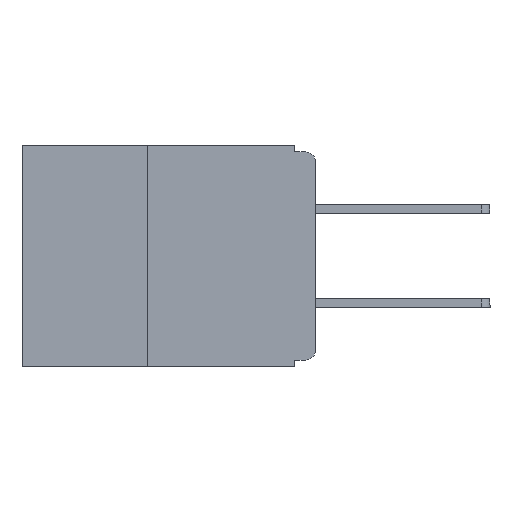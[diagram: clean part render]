
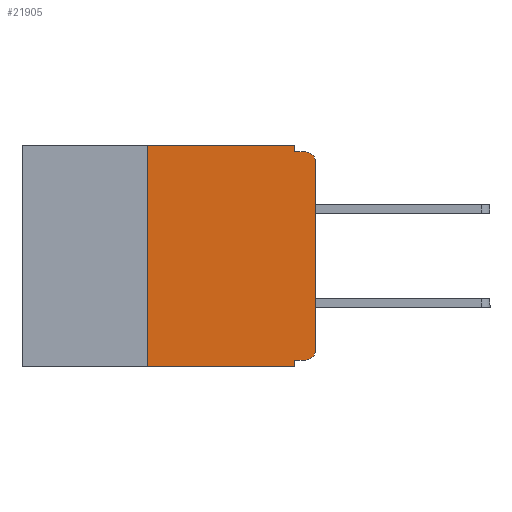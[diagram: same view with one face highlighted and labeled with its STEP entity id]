
A CAD part, left-side view. The second image highlights one B-rep face of the part: STEP entity #21905.
In plain terms, the highlighted planar face has unit normal (-1, 0, 0).
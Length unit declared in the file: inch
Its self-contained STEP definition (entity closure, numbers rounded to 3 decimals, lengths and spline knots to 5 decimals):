
#54 = VERTEX_POINT ( 'NONE', #20621 ) ;
#74 = CARTESIAN_POINT ( 'NONE',  ( 0., 0.015, -0.01 ) ) ;
#145 = DIRECTION ( 'NONE',  ( 0., 0., -1. ) ) ;
#631 = EDGE_CURVE ( 'NONE', #20836, #54, #11247, .T. ) ;
#1115 = DIRECTION ( 'NONE',  ( 0., 0., -1. ) ) ;
#1721 = CARTESIAN_POINT ( 'NONE',  ( 0., 0., -0.305 ) ) ;
#1859 = EDGE_CURVE ( 'NONE', #20836, #8800, #3649, .T. ) ;
#2239 = ORIENTED_EDGE ( 'NONE', *, *, #2959, .T. ) ;
#2360 = VERTEX_POINT ( 'NONE', #6417 ) ;
#2500 = EDGE_CURVE ( 'NONE', #19193, #18894, #23013, .T. ) ;
#2959 = EDGE_CURVE ( 'NONE', #10055, #19193, #12592, .T. ) ;
#3253 = LINE ( 'NONE', #12528, #17478 ) ;
#3649 = LINE ( 'NONE', #22574, #8000 ) ;
#4274 = DIRECTION ( 'NONE',  ( 0., 0., -1. ) ) ;
#4280 = ORIENTED_EDGE ( 'NONE', *, *, #5150, .F. ) ;
#5150 = EDGE_CURVE ( 'NONE', #8800, #2360, #15386, .T. ) ;
#5443 = ORIENTED_EDGE ( 'NONE', *, *, #631, .T. ) ;
#5676 = CARTESIAN_POINT ( 'NONE',  ( 0., 0.015, -0.32 ) ) ;
#5881 = CIRCLE ( 'NONE', #22462, 0.015 ) ;
#6032 = DIRECTION ( 'NONE',  ( -1., 0., 0. ) ) ;
#6249 = CARTESIAN_POINT ( 'NONE',  ( 0., 0.031, -0.32 ) ) ;
#6417 = CARTESIAN_POINT ( 'NONE',  ( 0., 0.031, 0. ) ) ;
#7265 = CARTESIAN_POINT ( 'NONE',  ( 0., 0., 0. ) ) ;
#7619 = CARTESIAN_POINT ( 'NONE',  ( 0., 0.031, -0.01 ) ) ;
#8000 = VECTOR ( 'NONE', #19025, 39.37008 ) ;
#8083 = EDGE_CURVE ( 'NONE', #2360, #8087, #19315, .T. ) ;
#8087 = VERTEX_POINT ( 'NONE', #7619 ) ;
#8090 = DIRECTION ( 'NONE',  ( 0., 0., -1. ) ) ;
#8601 = ORIENTED_EDGE ( 'NONE', *, *, #8083, .F. ) ;
#8800 = VERTEX_POINT ( 'NONE', #20902 ) ;
#9126 = LINE ( 'NONE', #19244, #14672 ) ;
#9141 = EDGE_CURVE ( 'NONE', #18894, #17457, #5881, .T. ) ;
#9349 = PLANE ( 'NONE',  #19904 ) ;
#9393 = VECTOR ( 'NONE', #20606, 39.37008 ) ;
#10055 = VERTEX_POINT ( 'NONE', #5676 ) ;
#10133 = LINE ( 'NONE', #14976, #18890 ) ;
#10362 = ORIENTED_EDGE ( 'NONE', *, *, #23383, .F. ) ;
#10857 = DIRECTION ( 'NONE',  ( 0., -1., 0. ) ) ;
#10966 = CARTESIAN_POINT ( 'NONE',  ( 0., 0.437, 0. ) ) ;
#10995 = DIRECTION ( 'NONE',  ( 0., -1., 0. ) ) ;
#11222 = ORIENTED_EDGE ( 'NONE', *, *, #2500, .T. ) ;
#11232 = DIRECTION ( 'NONE',  ( 1., 0., 0. ) ) ;
#11247 = LINE ( 'NONE', #16709, #21153 ) ;
#11530 = ORIENTED_EDGE ( 'NONE', *, *, #12920, .F. ) ;
#11850 = FACE_OUTER_BOUND ( 'NONE', #18250, .T. ) ;
#12202 = DIRECTION ( 'NONE',  ( -1., 0., 0. ) ) ;
#12528 = CARTESIAN_POINT ( 'NONE',  ( 0., 0., -0.01 ) ) ;
#12592 = CIRCLE ( 'NONE', #17275, 0.015 ) ;
#12920 = EDGE_CURVE ( 'NONE', #10055, #19437, #10133, .T. ) ;
#14135 = ORIENTED_EDGE ( 'NONE', *, *, #1859, .F. ) ;
#14351 = DIRECTION ( 'NONE',  ( 0., 0., 1. ) ) ;
#14672 = VECTOR ( 'NONE', #8090, 39.37008 ) ;
#14976 = CARTESIAN_POINT ( 'NONE',  ( 0., 0., -0.32 ) ) ;
#15386 = LINE ( 'NONE', #10966, #19188 ) ;
#15934 = CARTESIAN_POINT ( 'NONE',  ( 0., 0.015, -0.305 ) ) ;
#16709 = CARTESIAN_POINT ( 'NONE',  ( 0., 0.437, -0.33 ) ) ;
#16769 = DIRECTION ( 'NONE',  ( 0., 1., 0. ) ) ;
#17129 = CARTESIAN_POINT ( 'NONE',  ( 0., 0.25, -0.33 ) ) ;
#17275 = AXIS2_PLACEMENT_3D ( 'NONE', #15934, #6032, #4274 ) ;
#17457 = VERTEX_POINT ( 'NONE', #74 ) ;
#17478 = VECTOR ( 'NONE', #21855, 39.37008 ) ;
#18139 = VECTOR ( 'NONE', #14351, 39.37008 ) ;
#18250 = EDGE_LOOP ( 'NONE', ( #11222, #21686, #22810, #8601, #4280, #14135, #5443, #10362, #11530, #2239 ) ) ;
#18890 = VECTOR ( 'NONE', #16769, 39.37008 ) ;
#18894 = VERTEX_POINT ( 'NONE', #19352 ) ;
#19025 = DIRECTION ( 'NONE',  ( 0., 0., 1. ) ) ;
#19188 = VECTOR ( 'NONE', #10995, 39.37008 ) ;
#19193 = VERTEX_POINT ( 'NONE', #1721 ) ;
#19244 = CARTESIAN_POINT ( 'NONE',  ( 0., 0.031, -0.33 ) ) ;
#19315 = LINE ( 'NONE', #22429, #9393 ) ;
#19352 = CARTESIAN_POINT ( 'NONE',  ( 0., 0., -0.025 ) ) ;
#19437 = VERTEX_POINT ( 'NONE', #6249 ) ;
#19904 = AXIS2_PLACEMENT_3D ( 'NONE', #22329, #11232, #145 ) ;
#20389 = EDGE_CURVE ( 'NONE', #8087, #17457, #3253, .T. ) ;
#20606 = DIRECTION ( 'NONE',  ( 0., 0., -1. ) ) ;
#20621 = CARTESIAN_POINT ( 'NONE',  ( 0., 0.031, -0.33 ) ) ;
#20836 = VERTEX_POINT ( 'NONE', #17129 ) ;
#20902 = CARTESIAN_POINT ( 'NONE',  ( 0., 0.25, 0. ) ) ;
#21153 = VECTOR ( 'NONE', #10857, 39.37008 ) ;
#21686 = ORIENTED_EDGE ( 'NONE', *, *, #9141, .T. ) ;
#21855 = DIRECTION ( 'NONE',  ( 0., -1., 0. ) ) ;
#21905 = ADVANCED_FACE ( 'NONE', ( #11850 ), #9349, .F. ) ;
#22329 = CARTESIAN_POINT ( 'NONE',  ( 0., 0.437, 0. ) ) ;
#22429 = CARTESIAN_POINT ( 'NONE',  ( 0., 0.031, 0. ) ) ;
#22462 = AXIS2_PLACEMENT_3D ( 'NONE', #23267, #12202, #1115 ) ;
#22574 = CARTESIAN_POINT ( 'NONE',  ( 0., 0.25, -0.33 ) ) ;
#22810 = ORIENTED_EDGE ( 'NONE', *, *, #20389, .F. ) ;
#23013 = LINE ( 'NONE', #7265, #18139 ) ;
#23267 = CARTESIAN_POINT ( 'NONE',  ( 0., 0.015, -0.025 ) ) ;
#23383 = EDGE_CURVE ( 'NONE', #19437, #54, #9126, .T. ) ;
